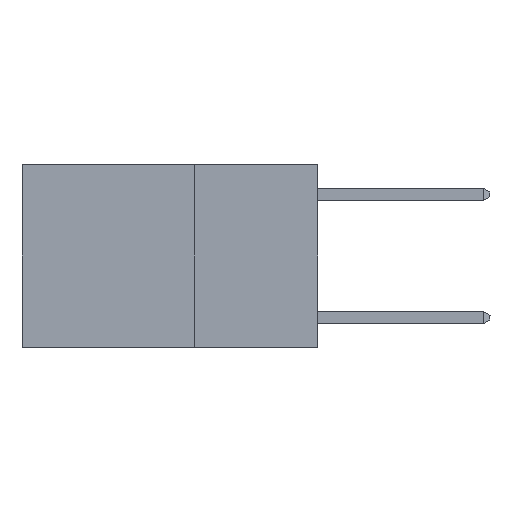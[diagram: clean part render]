
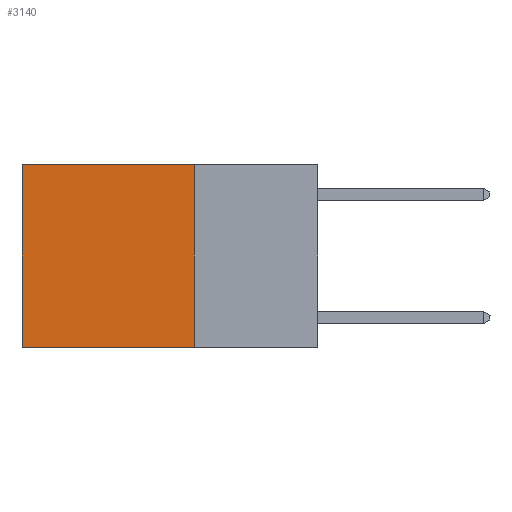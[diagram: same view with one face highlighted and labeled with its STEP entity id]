
A CAD part, left-side view. The second image highlights one B-rep face of the part: STEP entity #3140.
In plain terms, the highlighted planar face has unit normal (-1, 0, 0).
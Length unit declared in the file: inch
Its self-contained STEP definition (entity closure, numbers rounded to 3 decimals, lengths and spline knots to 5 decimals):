
#230 = AXIS2_PLACEMENT_3D ( 'NONE', #10605, #652, #6768 ) ;
#354 = EDGE_CURVE ( 'NONE', #4087, #10217, #7091, .T. ) ;
#413 = VECTOR ( 'NONE', #1404, 39.37008 ) ;
#652 = DIRECTION ( 'NONE',  ( 1., 0., 0. ) ) ;
#1404 = DIRECTION ( 'NONE',  ( 0., 1., 0. ) ) ;
#1548 = DIRECTION ( 'NONE',  ( 0., 0., -1. ) ) ;
#1897 = VECTOR ( 'NONE', #3667, 39.37008 ) ;
#2085 = DIRECTION ( 'NONE',  ( 0., 1., 0. ) ) ;
#2208 = FACE_OUTER_BOUND ( 'NONE', #8895, .T. ) ;
#2620 = VECTOR ( 'NONE', #1548, 39.37008 ) ;
#3140 = ADVANCED_FACE ( 'NONE', ( #2208 ), #10638, .F. ) ;
#3225 = VERTEX_POINT ( 'NONE', #6898 ) ;
#3423 = ORIENTED_EDGE ( 'NONE', *, *, #354, .F. ) ;
#3579 = EDGE_CURVE ( 'NONE', #6571, #10217, #9264, .T. ) ;
#3667 = DIRECTION ( 'NONE',  ( 0., 0., -1. ) ) ;
#3771 = EDGE_CURVE ( 'NONE', #3225, #4087, #10691, .T. ) ;
#3814 = ORIENTED_EDGE ( 'NONE', *, *, #3579, .T. ) ;
#4087 = VERTEX_POINT ( 'NONE', #5676 ) ;
#4201 = VECTOR ( 'NONE', #2085, 39.37008 ) ;
#4209 = CARTESIAN_POINT ( 'NONE',  ( 0.2625, 0.6, 0. ) ) ;
#5628 = ORIENTED_EDGE ( 'NONE', *, *, #3771, .F. ) ;
#5676 = CARTESIAN_POINT ( 'NONE',  ( 0.2625, 0.25, -0.37 ) ) ;
#5938 = CARTESIAN_POINT ( 'NONE',  ( 0.2625, 0.6, -0.37 ) ) ;
#5962 = CARTESIAN_POINT ( 'NONE',  ( 0.2625, 0.25, -0.37 ) ) ;
#6571 = VERTEX_POINT ( 'NONE', #6838 ) ;
#6768 = DIRECTION ( 'NONE',  ( 0., 0., -1. ) ) ;
#6838 = CARTESIAN_POINT ( 'NONE',  ( 0.2625, 0.6, 0. ) ) ;
#6898 = CARTESIAN_POINT ( 'NONE',  ( 0.2625, 0.25, 0. ) ) ;
#7091 = LINE ( 'NONE', #5962, #413 ) ;
#7329 = EDGE_CURVE ( 'NONE', #3225, #6571, #10642, .T. ) ;
#7842 = ORIENTED_EDGE ( 'NONE', *, *, #7329, .T. ) ;
#8064 = CARTESIAN_POINT ( 'NONE',  ( 0.2625, 0.25, 0. ) ) ;
#8651 = CARTESIAN_POINT ( 'NONE',  ( 0.2625, 0.25, 0. ) ) ;
#8895 = EDGE_LOOP ( 'NONE', ( #3814, #3423, #5628, #7842 ) ) ;
#9264 = LINE ( 'NONE', #4209, #2620 ) ;
#10217 = VERTEX_POINT ( 'NONE', #5938 ) ;
#10605 = CARTESIAN_POINT ( 'NONE',  ( 0.2625, 0.25, 0. ) ) ;
#10638 = PLANE ( 'NONE',  #230 ) ;
#10642 = LINE ( 'NONE', #8064, #4201 ) ;
#10691 = LINE ( 'NONE', #8651, #1897 ) ;
